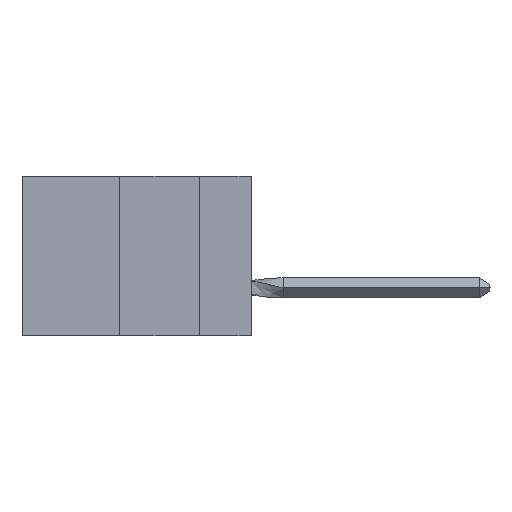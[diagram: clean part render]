
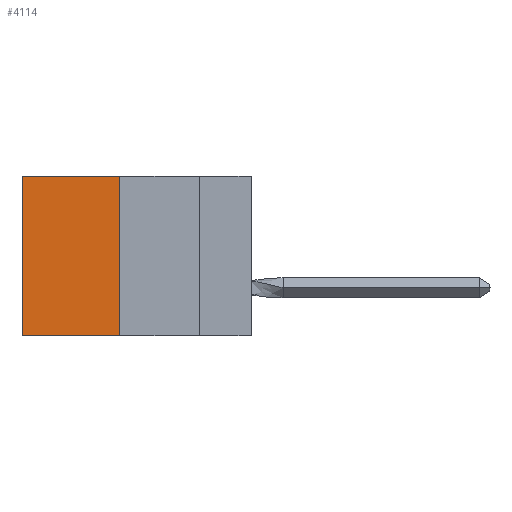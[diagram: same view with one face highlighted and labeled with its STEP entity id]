
A CAD part, left-side view. The second image highlights one B-rep face of the part: STEP entity #4114.
In plain terms, the highlighted planar face has unit normal (-1, 0, 0).
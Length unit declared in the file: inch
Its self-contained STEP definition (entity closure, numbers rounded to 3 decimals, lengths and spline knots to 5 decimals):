
#488 = DIRECTION ( 'NONE',  ( 0., 0., -1. ) ) ;
#1662 = EDGE_LOOP ( 'NONE', ( #21679, #15020, #24177, #28602 ) ) ;
#2190 = CARTESIAN_POINT ( 'NONE',  ( 0.305, 0.413, -0.5 ) ) ;
#3105 = DIRECTION ( 'NONE',  ( 0., 1., 0. ) ) ;
#3272 = CARTESIAN_POINT ( 'NONE',  ( 0.305, 0.72, 0. ) ) ;
#3405 = VECTOR ( 'NONE', #9121, 39.37008 ) ;
#4114 = ADVANCED_FACE ( 'NONE', ( #30769 ), #21404, .F. ) ;
#4893 = EDGE_CURVE ( 'NONE', #17405, #24365, #31136, .T. ) ;
#5713 = LINE ( 'NONE', #14445, #22904 ) ;
#6654 = VECTOR ( 'NONE', #488, 39.37008 ) ;
#6940 = CARTESIAN_POINT ( 'NONE',  ( 0.305, 0.72, -0.5 ) ) ;
#9121 = DIRECTION ( 'NONE',  ( 0., 1., 0. ) ) ;
#10658 = LINE ( 'NONE', #6940, #25941 ) ;
#11260 = EDGE_CURVE ( 'NONE', #24365, #13020, #30109, .T. ) ;
#13020 = VERTEX_POINT ( 'NONE', #27297 ) ;
#13963 = CARTESIAN_POINT ( 'NONE',  ( 0.305, 0.413, -0.5 ) ) ;
#14071 = DIRECTION ( 'NONE',  ( 1., 0., 0. ) ) ;
#14368 = CARTESIAN_POINT ( 'NONE',  ( 0.305, 0.413, -0.5 ) ) ;
#14369 = EDGE_CURVE ( 'NONE', #16192, #13020, #10658, .T. ) ;
#14445 = CARTESIAN_POINT ( 'NONE',  ( 0.305, 0.413, 0. ) ) ;
#15020 = ORIENTED_EDGE ( 'NONE', *, *, #11260, .F. ) ;
#15393 = CARTESIAN_POINT ( 'NONE',  ( 0.305, 0.413, -0.5 ) ) ;
#16192 = VERTEX_POINT ( 'NONE', #3272 ) ;
#16803 = DIRECTION ( 'NONE',  ( 0., 0., -1. ) ) ;
#17405 = VERTEX_POINT ( 'NONE', #28410 ) ;
#18310 = EDGE_CURVE ( 'NONE', #17405, #16192, #5713, .T. ) ;
#20655 = AXIS2_PLACEMENT_3D ( 'NONE', #14368, #14071, #31131 ) ;
#21404 = PLANE ( 'NONE',  #20655 ) ;
#21679 = ORIENTED_EDGE ( 'NONE', *, *, #14369, .T. ) ;
#22904 = VECTOR ( 'NONE', #3105, 39.37008 ) ;
#24177 = ORIENTED_EDGE ( 'NONE', *, *, #4893, .F. ) ;
#24365 = VERTEX_POINT ( 'NONE', #13963 ) ;
#25941 = VECTOR ( 'NONE', #16803, 39.37008 ) ;
#27297 = CARTESIAN_POINT ( 'NONE',  ( 0.305, 0.72, -0.5 ) ) ;
#28410 = CARTESIAN_POINT ( 'NONE',  ( 0.305, 0.413, 0. ) ) ;
#28602 = ORIENTED_EDGE ( 'NONE', *, *, #18310, .T. ) ;
#30109 = LINE ( 'NONE', #2190, #3405 ) ;
#30769 = FACE_OUTER_BOUND ( 'NONE', #1662, .T. ) ;
#31131 = DIRECTION ( 'NONE',  ( 0., 0., -1. ) ) ;
#31136 = LINE ( 'NONE', #15393, #6654 ) ;
